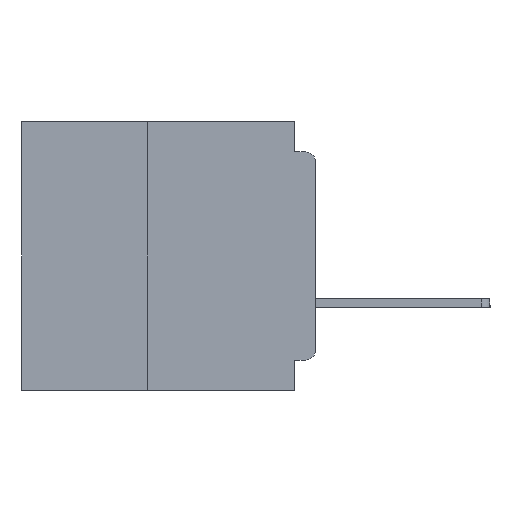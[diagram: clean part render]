
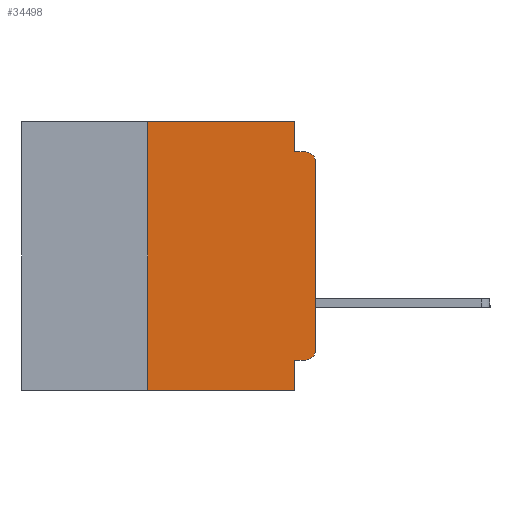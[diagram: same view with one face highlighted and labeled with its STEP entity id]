
A CAD part, left-side view. The second image highlights one B-rep face of the part: STEP entity #34498.
In plain terms, the highlighted planar face has unit normal (-1, 0, 0).
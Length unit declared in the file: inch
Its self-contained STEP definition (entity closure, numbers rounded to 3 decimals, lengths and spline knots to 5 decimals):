
#520 = LINE ( 'NONE', #4985, #8338 ) ;
#1628 = DIRECTION ( 'NONE',  ( 0., -1., 0. ) ) ;
#1846 = VERTEX_POINT ( 'NONE', #19212 ) ;
#3662 = EDGE_CURVE ( 'NONE', #35100, #40086, #26998, .T. ) ;
#3952 = EDGE_CURVE ( 'NONE', #5468, #1846, #31083, .T. ) ;
#4375 = ORIENTED_EDGE ( 'NONE', *, *, #22348, .T. ) ;
#4894 = LINE ( 'NONE', #16833, #12658 ) ;
#4985 = CARTESIAN_POINT ( 'NONE',  ( 0., 0.437, 0. ) ) ;
#5468 = VERTEX_POINT ( 'NONE', #6797 ) ;
#5502 = ORIENTED_EDGE ( 'NONE', *, *, #41210, .T. ) ;
#5503 = CARTESIAN_POINT ( 'NONE',  ( 0., 0.437, 0. ) ) ;
#5591 = CARTESIAN_POINT ( 'NONE',  ( 0., 0.015, -0.34 ) ) ;
#6797 = CARTESIAN_POINT ( 'NONE',  ( 0., 0.031, 0. ) ) ;
#7206 = EDGE_CURVE ( 'NONE', #1846, #29953, #15024, .T. ) ;
#8338 = VECTOR ( 'NONE', #1628, 39.37008 ) ;
#8502 = ORIENTED_EDGE ( 'NONE', *, *, #3662, .F. ) ;
#8650 = DIRECTION ( 'NONE',  ( 0., 0., 1. ) ) ;
#8942 = DIRECTION ( 'NONE',  ( 0., 0., -1. ) ) ;
#9098 = EDGE_CURVE ( 'NONE', #40086, #16455, #22484, .T. ) ;
#9352 = VERTEX_POINT ( 'NONE', #23035 ) ;
#10199 = CARTESIAN_POINT ( 'NONE',  ( 0., 0.015, -0.045 ) ) ;
#10528 = VERTEX_POINT ( 'NONE', #36322 ) ;
#10800 = AXIS2_PLACEMENT_3D ( 'NONE', #31957, #12475, #35207 ) ;
#12265 = CARTESIAN_POINT ( 'NONE',  ( 0., 0.031, 0. ) ) ;
#12475 = DIRECTION ( 'NONE',  ( -1., 0., 0. ) ) ;
#12658 = VECTOR ( 'NONE', #20083, 39.37008 ) ;
#12844 = CARTESIAN_POINT ( 'NONE',  ( 0., 0., -0.045 ) ) ;
#13786 = VECTOR ( 'NONE', #15517, 39.37008 ) ;
#13796 = ORIENTED_EDGE ( 'NONE', *, *, #36005, .F. ) ;
#14314 = VECTOR ( 'NONE', #8650, 39.37008 ) ;
#15024 = LINE ( 'NONE', #12844, #39896 ) ;
#15335 = FACE_OUTER_BOUND ( 'NONE', #17122, .T. ) ;
#15517 = DIRECTION ( 'NONE',  ( 0., 0., -1. ) ) ;
#15730 = CARTESIAN_POINT ( 'NONE',  ( 0., 0., -0.06 ) ) ;
#16044 = ORIENTED_EDGE ( 'NONE', *, *, #7206, .F. ) ;
#16101 = DIRECTION ( 'NONE',  ( 0., -1., 0. ) ) ;
#16455 = VERTEX_POINT ( 'NONE', #35781 ) ;
#16833 = CARTESIAN_POINT ( 'NONE',  ( 0., 0.25, -0.4 ) ) ;
#17122 = EDGE_LOOP ( 'NONE', ( #5502, #19248, #16044, #34111, #27586, #13796, #24240, #40699, #8502, #4375 ) ) ;
#18663 = DIRECTION ( 'NONE',  ( 0., 0., -1. ) ) ;
#18729 = CARTESIAN_POINT ( 'NONE',  ( 0., 0.25, 0. ) ) ;
#19212 = CARTESIAN_POINT ( 'NONE',  ( 0., 0.031, -0.045 ) ) ;
#19248 = ORIENTED_EDGE ( 'NONE', *, *, #35816, .T. ) ;
#20083 = DIRECTION ( 'NONE',  ( 0., 0., 1. ) ) ;
#20348 = CARTESIAN_POINT ( 'NONE',  ( 0., 0., -0.355 ) ) ;
#22333 = LINE ( 'NONE', #34561, #14314 ) ;
#22348 = EDGE_CURVE ( 'NONE', #35100, #9352, #25166, .T. ) ;
#22484 = LINE ( 'NONE', #28200, #29135 ) ;
#22994 = EDGE_CURVE ( 'NONE', #24897, #5468, #520, .T. ) ;
#23035 = CARTESIAN_POINT ( 'NONE',  ( 0., 0., -0.34 ) ) ;
#23541 = EDGE_CURVE ( 'NONE', #10528, #16455, #23557, .T. ) ;
#23557 = LINE ( 'NONE', #31095, #31225 ) ;
#24240 = ORIENTED_EDGE ( 'NONE', *, *, #23541, .T. ) ;
#24506 = DIRECTION ( 'NONE',  ( 0., -1., 0. ) ) ;
#24897 = VERTEX_POINT ( 'NONE', #18729 ) ;
#25037 = DIRECTION ( 'NONE',  ( 0., 0., -1. ) ) ;
#25166 = CIRCLE ( 'NONE', #36122, 0.015 ) ;
#26998 = LINE ( 'NONE', #20348, #34667 ) ;
#27586 = ORIENTED_EDGE ( 'NONE', *, *, #22994, .F. ) ;
#28200 = CARTESIAN_POINT ( 'NONE',  ( 0., 0.031, -0.4 ) ) ;
#28436 = DIRECTION ( 'NONE',  ( -1., 0., 0. ) ) ;
#28825 = CARTESIAN_POINT ( 'NONE',  ( 0., 0.031, -0.355 ) ) ;
#29135 = VECTOR ( 'NONE', #25037, 39.37008 ) ;
#29953 = VERTEX_POINT ( 'NONE', #10199 ) ;
#30471 = CIRCLE ( 'NONE', #10800, 0.015 ) ;
#31083 = LINE ( 'NONE', #12265, #13786 ) ;
#31095 = CARTESIAN_POINT ( 'NONE',  ( 0., 0.437, -0.4 ) ) ;
#31225 = VECTOR ( 'NONE', #24506, 39.37008 ) ;
#31957 = CARTESIAN_POINT ( 'NONE',  ( 0., 0.015, -0.06 ) ) ;
#34111 = ORIENTED_EDGE ( 'NONE', *, *, #3952, .F. ) ;
#34441 = AXIS2_PLACEMENT_3D ( 'NONE', #5503, #38115, #18663 ) ;
#34498 = ADVANCED_FACE ( 'NONE', ( #15335 ), #34880, .F. ) ;
#34561 = CARTESIAN_POINT ( 'NONE',  ( 0., 0., 0. ) ) ;
#34667 = VECTOR ( 'NONE', #39826, 39.37008 ) ;
#34697 = CARTESIAN_POINT ( 'NONE',  ( 0., 0.015, -0.355 ) ) ;
#34880 = PLANE ( 'NONE',  #34441 ) ;
#35100 = VERTEX_POINT ( 'NONE', #34697 ) ;
#35207 = DIRECTION ( 'NONE',  ( 0., 0., -1. ) ) ;
#35781 = CARTESIAN_POINT ( 'NONE',  ( 0., 0.031, -0.4 ) ) ;
#35816 = EDGE_CURVE ( 'NONE', #35838, #29953, #30471, .T. ) ;
#35838 = VERTEX_POINT ( 'NONE', #15730 ) ;
#36005 = EDGE_CURVE ( 'NONE', #10528, #24897, #4894, .T. ) ;
#36122 = AXIS2_PLACEMENT_3D ( 'NONE', #5591, #28436, #8942 ) ;
#36322 = CARTESIAN_POINT ( 'NONE',  ( 0., 0.25, -0.4 ) ) ;
#38115 = DIRECTION ( 'NONE',  ( 1., 0., 0. ) ) ;
#39826 = DIRECTION ( 'NONE',  ( 0., 1., 0. ) ) ;
#39896 = VECTOR ( 'NONE', #16101, 39.37008 ) ;
#40086 = VERTEX_POINT ( 'NONE', #28825 ) ;
#40699 = ORIENTED_EDGE ( 'NONE', *, *, #9098, .F. ) ;
#41210 = EDGE_CURVE ( 'NONE', #9352, #35838, #22333, .T. ) ;
